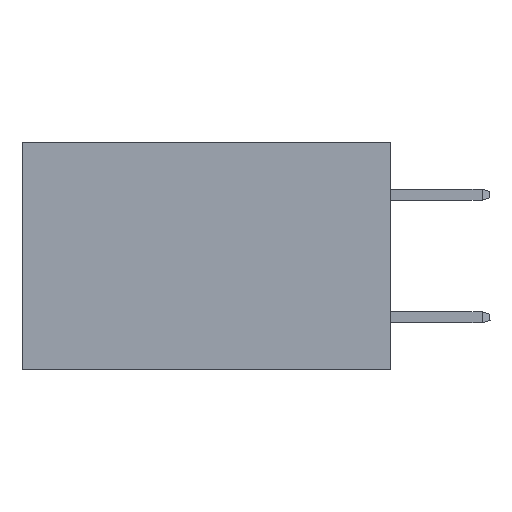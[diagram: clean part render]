
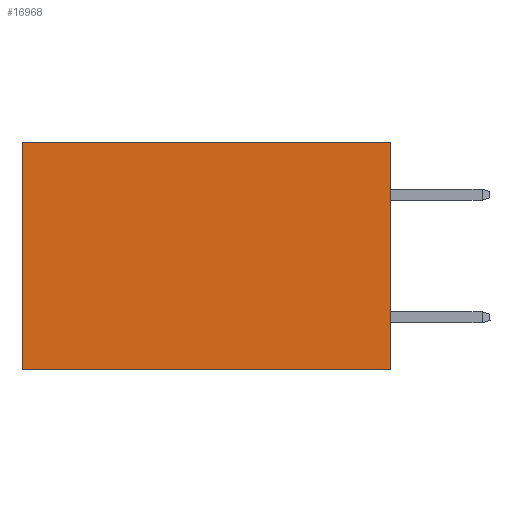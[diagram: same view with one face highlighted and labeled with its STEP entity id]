
A CAD part, left-side view. The second image highlights one B-rep face of the part: STEP entity #16968.
In plain terms, the highlighted planar face has unit normal (-1, 0, 0).
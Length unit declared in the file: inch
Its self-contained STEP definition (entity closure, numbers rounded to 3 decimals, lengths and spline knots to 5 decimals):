
#630 = PLANE ( 'NONE',  #18932 ) ;
#1528 = VECTOR ( 'NONE', #27329, 39.37008 ) ;
#3373 = DIRECTION ( 'NONE',  ( 0., 0., -1. ) ) ;
#5422 = DIRECTION ( 'NONE',  ( 1., 0., 0. ) ) ;
#5662 = EDGE_CURVE ( 'NONE', #19144, #11512, #6189, .T. ) ;
#6189 = LINE ( 'NONE', #22988, #1528 ) ;
#8430 = EDGE_CURVE ( 'NONE', #10958, #11955, #10047, .T. ) ;
#10047 = LINE ( 'NONE', #20751, #21838 ) ;
#10958 = VERTEX_POINT ( 'NONE', #13966 ) ;
#11512 = VERTEX_POINT ( 'NONE', #20369 ) ;
#11603 = FACE_OUTER_BOUND ( 'NONE', #15157, .T. ) ;
#11955 = VERTEX_POINT ( 'NONE', #18401 ) ;
#13774 = ORIENTED_EDGE ( 'NONE', *, *, #24363, .F. ) ;
#13966 = CARTESIAN_POINT ( 'NONE',  ( 0.2875, 0., -0.37 ) ) ;
#15157 = EDGE_LOOP ( 'NONE', ( #24145, #20587, #13774, #19205 ) ) ;
#16968 = ADVANCED_FACE ( 'NONE', ( #11603 ), #630, .F. ) ;
#18401 = CARTESIAN_POINT ( 'NONE',  ( 0.2875, 0.6, -0.37 ) ) ;
#18932 = AXIS2_PLACEMENT_3D ( 'NONE', #21218, #5422, #21413 ) ;
#19144 = VERTEX_POINT ( 'NONE', #28215 ) ;
#19205 = ORIENTED_EDGE ( 'NONE', *, *, #5662, .T. ) ;
#20369 = CARTESIAN_POINT ( 'NONE',  ( 0.2875, 0.6, 0. ) ) ;
#20587 = ORIENTED_EDGE ( 'NONE', *, *, #8430, .F. ) ;
#20751 = CARTESIAN_POINT ( 'NONE',  ( 0.2875, 0., -0.37 ) ) ;
#20854 = DIRECTION ( 'NONE',  ( 0., 1., 0. ) ) ;
#21218 = CARTESIAN_POINT ( 'NONE',  ( 0.2875, 0., 0. ) ) ;
#21413 = DIRECTION ( 'NONE',  ( 0., 0., -1. ) ) ;
#21838 = VECTOR ( 'NONE', #20854, 39.37008 ) ;
#22914 = VECTOR ( 'NONE', #3373, 39.37008 ) ;
#22988 = CARTESIAN_POINT ( 'NONE',  ( 0.2875, 0., 0. ) ) ;
#23242 = LINE ( 'NONE', #26075, #22914 ) ;
#24145 = ORIENTED_EDGE ( 'NONE', *, *, #28119, .T. ) ;
#24363 = EDGE_CURVE ( 'NONE', #19144, #10958, #23242, .T. ) ;
#24942 = VECTOR ( 'NONE', #28783, 39.37008 ) ;
#26075 = CARTESIAN_POINT ( 'NONE',  ( 0.2875, 0., 0. ) ) ;
#26503 = CARTESIAN_POINT ( 'NONE',  ( 0.2875, 0.6, 0. ) ) ;
#26717 = LINE ( 'NONE', #26503, #24942 ) ;
#27329 = DIRECTION ( 'NONE',  ( 0., 1., 0. ) ) ;
#28119 = EDGE_CURVE ( 'NONE', #11512, #11955, #26717, .T. ) ;
#28215 = CARTESIAN_POINT ( 'NONE',  ( 0.2875, 0., 0. ) ) ;
#28783 = DIRECTION ( 'NONE',  ( 0., 0., -1. ) ) ;
